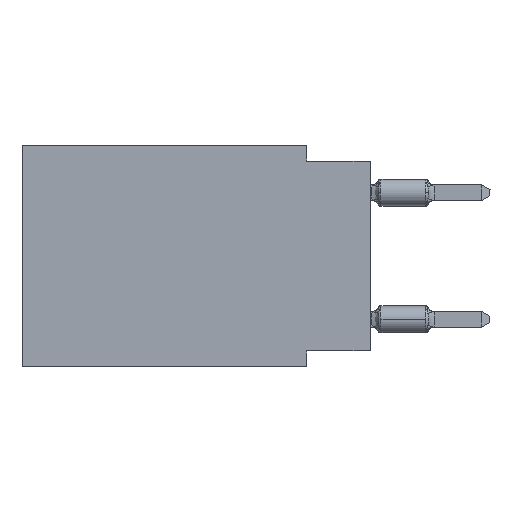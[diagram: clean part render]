
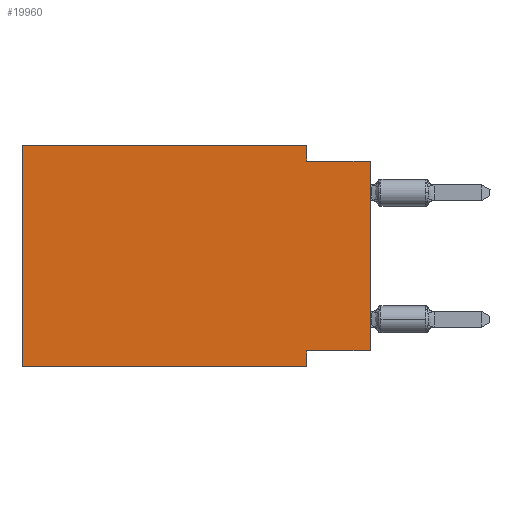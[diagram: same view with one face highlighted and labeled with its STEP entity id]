
A CAD part, left-side view. The second image highlights one B-rep face of the part: STEP entity #19960.
In plain terms, the highlighted planar face has unit normal (-1, 0, 0).
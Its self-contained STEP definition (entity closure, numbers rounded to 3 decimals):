
#248 = CARTESIAN_POINT ( 'NONE',  ( 0., 2.54, -8.89 ) ) ;
#485 = VERTEX_POINT ( 'NONE', #18077 ) ;
#1034 = CARTESIAN_POINT ( 'NONE',  ( 0., 2.54, 0. ) ) ;
#1147 = VECTOR ( 'NONE', #20992, 1000. ) ;
#1529 = VECTOR ( 'NONE', #2211, 1000. ) ;
#1670 = VERTEX_POINT ( 'NONE', #11370 ) ;
#1730 = VERTEX_POINT ( 'NONE', #2050 ) ;
#2050 = CARTESIAN_POINT ( 'NONE',  ( 0., 0., -8.255 ) ) ;
#2211 = DIRECTION ( 'NONE',  ( 0., -1., 0. ) ) ;
#2712 = DIRECTION ( 'NONE',  ( 0., -1., 0. ) ) ;
#2962 = VERTEX_POINT ( 'NONE', #20507 ) ;
#2963 = ORIENTED_EDGE ( 'NONE', *, *, #9098, .T. ) ;
#3131 = LINE ( 'NONE', #18182, #19281 ) ;
#3317 = DIRECTION ( 'NONE',  ( 0., 0., -1. ) ) ;
#3658 = DIRECTION ( 'NONE',  ( 0., 0., 1. ) ) ;
#3842 = DIRECTION ( 'NONE',  ( 0., -1., 0. ) ) ;
#4247 = EDGE_CURVE ( 'NONE', #1670, #485, #21010, .T. ) ;
#4895 = VECTOR ( 'NONE', #3842, 1000. ) ;
#5390 = ORIENTED_EDGE ( 'NONE', *, *, #7842, .F. ) ;
#5391 = EDGE_CURVE ( 'NONE', #1730, #485, #5542, .T. ) ;
#5542 = LINE ( 'NONE', #11511, #1147 ) ;
#5887 = LINE ( 'NONE', #13488, #11242 ) ;
#5914 = VECTOR ( 'NONE', #3317, 1000. ) ;
#6139 = EDGE_CURVE ( 'NONE', #1730, #24520, #14711, .T. ) ;
#6177 = CARTESIAN_POINT ( 'NONE',  ( 0., 13.97, -8.89 ) ) ;
#7045 = EDGE_CURVE ( 'NONE', #8692, #2962, #5887, .T. ) ;
#7538 = CARTESIAN_POINT ( 'NONE',  ( 0., 2.54, 0. ) ) ;
#7576 = AXIS2_PLACEMENT_3D ( 'NONE', #16954, #15083, #11220 ) ;
#7842 = EDGE_CURVE ( 'NONE', #2962, #21938, #22786, .T. ) ;
#8445 = ORIENTED_EDGE ( 'NONE', *, *, #7045, .F. ) ;
#8692 = VERTEX_POINT ( 'NONE', #14971 ) ;
#8971 = DIRECTION ( 'NONE',  ( 0., 0., -1. ) ) ;
#9098 = EDGE_CURVE ( 'NONE', #8692, #17035, #11902, .T. ) ;
#9328 = EDGE_CURVE ( 'NONE', #24520, #17035, #3131, .T. ) ;
#9912 = CARTESIAN_POINT ( 'NONE',  ( 0., 0., -0.635 ) ) ;
#10512 = VECTOR ( 'NONE', #2712, 1000. ) ;
#11220 = DIRECTION ( 'NONE',  ( 0., 0., -1. ) ) ;
#11242 = VECTOR ( 'NONE', #3658, 1000. ) ;
#11334 = DIRECTION ( 'NONE',  ( 0., 1., 0. ) ) ;
#11370 = CARTESIAN_POINT ( 'NONE',  ( 0., 2.54, -0.635 ) ) ;
#11455 = FACE_OUTER_BOUND ( 'NONE', #18927, .T. ) ;
#11511 = CARTESIAN_POINT ( 'NONE',  ( 0., 0., 0. ) ) ;
#11902 = LINE ( 'NONE', #6177, #10512 ) ;
#11989 = ORIENTED_EDGE ( 'NONE', *, *, #9328, .F. ) ;
#12475 = ORIENTED_EDGE ( 'NONE', *, *, #4247, .F. ) ;
#12936 = ORIENTED_EDGE ( 'NONE', *, *, #6139, .F. ) ;
#13303 = CARTESIAN_POINT ( 'NONE',  ( 0., 13.97, 0. ) ) ;
#13488 = CARTESIAN_POINT ( 'NONE',  ( 0., 13.97, 0. ) ) ;
#13624 = ORIENTED_EDGE ( 'NONE', *, *, #5391, .T. ) ;
#14711 = LINE ( 'NONE', #24451, #14795 ) ;
#14795 = VECTOR ( 'NONE', #11334, 1000. ) ;
#14899 = LINE ( 'NONE', #7538, #5914 ) ;
#14971 = CARTESIAN_POINT ( 'NONE',  ( 0., 13.97, -8.89 ) ) ;
#15083 = DIRECTION ( 'NONE',  ( 1., 0., 0. ) ) ;
#15960 = EDGE_CURVE ( 'NONE', #21938, #1670, #14899, .T. ) ;
#16954 = CARTESIAN_POINT ( 'NONE',  ( 0., 13.97, 0. ) ) ;
#17035 = VERTEX_POINT ( 'NONE', #248 ) ;
#18077 = CARTESIAN_POINT ( 'NONE',  ( 0., 0., -0.635 ) ) ;
#18182 = CARTESIAN_POINT ( 'NONE',  ( 0., 2.54, -8.89 ) ) ;
#18691 = PLANE ( 'NONE',  #7576 ) ;
#18927 = EDGE_LOOP ( 'NONE', ( #13624, #12475, #21090, #5390, #8445, #2963, #11989, #12936 ) ) ;
#19195 = CARTESIAN_POINT ( 'NONE',  ( 0., 2.54, -8.255 ) ) ;
#19281 = VECTOR ( 'NONE', #8971, 1000. ) ;
#19960 = ADVANCED_FACE ( 'NONE', ( #11455 ), #18691, .F. ) ;
#20507 = CARTESIAN_POINT ( 'NONE',  ( 0., 13.97, 0. ) ) ;
#20992 = DIRECTION ( 'NONE',  ( 0., 0., 1. ) ) ;
#21010 = LINE ( 'NONE', #9912, #1529 ) ;
#21090 = ORIENTED_EDGE ( 'NONE', *, *, #15960, .F. ) ;
#21938 = VERTEX_POINT ( 'NONE', #1034 ) ;
#22786 = LINE ( 'NONE', #13303, #4895 ) ;
#24451 = CARTESIAN_POINT ( 'NONE',  ( 0., 0., -8.255 ) ) ;
#24520 = VERTEX_POINT ( 'NONE', #19195 ) ;
